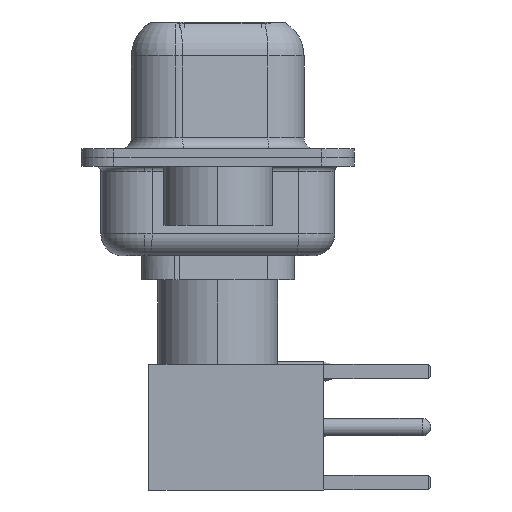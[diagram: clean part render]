
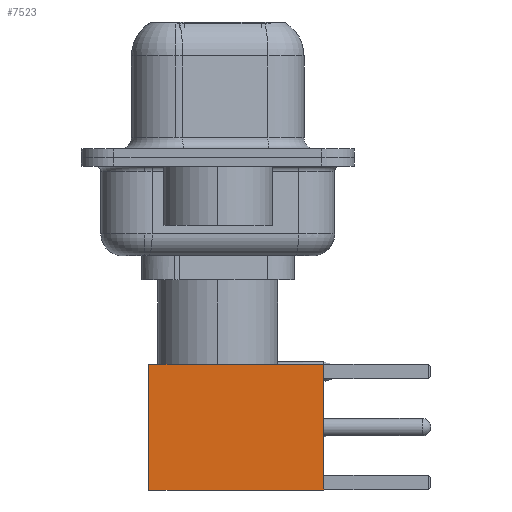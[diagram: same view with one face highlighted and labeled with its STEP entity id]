
A CAD part, left-side view. The second image highlights one B-rep face of the part: STEP entity #7523.
In plain terms, the highlighted face is planar.
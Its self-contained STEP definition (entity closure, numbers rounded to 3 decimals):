
#844 = CARTESIAN_POINT ( 'NONE',  ( -2.875, 2.875, 0. ) ) ;
#2040 = EDGE_CURVE ( 'NONE', #3056, #16021, #9995, .T. ) ;
#2336 = VERTEX_POINT ( 'NONE', #9125 ) ;
#2946 = PLANE ( 'NONE',  #22086 ) ;
#3056 = VERTEX_POINT ( 'NONE', #12006 ) ;
#3095 = LINE ( 'NONE', #12608, #9337 ) ;
#3867 = DIRECTION ( 'NONE',  ( -1., 0., 0. ) ) ;
#4305 = FACE_OUTER_BOUND ( 'NONE', #21728, .T. ) ;
#4921 = ORIENTED_EDGE ( 'NONE', *, *, #8052, .F. ) ;
#5228 = ORIENTED_EDGE ( 'NONE', *, *, #20506, .T. ) ;
#7199 = EDGE_CURVE ( 'NONE', #2336, #10379, #3095, .T. ) ;
#7523 = ADVANCED_FACE ( 'NONE', ( #4305 ), #2946, .T. ) ;
#8052 = EDGE_CURVE ( 'NONE', #2336, #3056, #12764, .T. ) ;
#9125 = CARTESIAN_POINT ( 'NONE',  ( 2.875, 2.875, 8. ) ) ;
#9154 = ORIENTED_EDGE ( 'NONE', *, *, #7199, .T. ) ;
#9337 = VECTOR ( 'NONE', #10874, 1000. ) ;
#9995 = LINE ( 'NONE', #10241, #19126 ) ;
#10241 = CARTESIAN_POINT ( 'NONE',  ( -2.875, 2.875, 0. ) ) ;
#10379 = VERTEX_POINT ( 'NONE', #16181 ) ;
#10874 = DIRECTION ( 'NONE',  ( 0., 0., -1. ) ) ;
#11281 = CARTESIAN_POINT ( 'NONE',  ( 0., 2.875, 0. ) ) ;
#12006 = CARTESIAN_POINT ( 'NONE',  ( -2.875, 2.875, 8. ) ) ;
#12340 = CARTESIAN_POINT ( 'NONE',  ( 2.875, 2.875, 0. ) ) ;
#12608 = CARTESIAN_POINT ( 'NONE',  ( 2.875, 2.875, 0. ) ) ;
#12764 = LINE ( 'NONE', #14883, #22501 ) ;
#14883 = CARTESIAN_POINT ( 'NONE',  ( 0., 2.875, 8. ) ) ;
#15005 = DIRECTION ( 'NONE',  ( -1., 0., 0. ) ) ;
#15679 = DIRECTION ( 'NONE',  ( 0., 0., -1. ) ) ;
#16021 = VERTEX_POINT ( 'NONE', #844 ) ;
#16181 = CARTESIAN_POINT ( 'NONE',  ( 2.875, 2.875, 0. ) ) ;
#17903 = DIRECTION ( 'NONE',  ( 0., 0., 1. ) ) ;
#18252 = VECTOR ( 'NONE', #3867, 1000. ) ;
#19126 = VECTOR ( 'NONE', #15679, 1000. ) ;
#20506 = EDGE_CURVE ( 'NONE', #10379, #16021, #24261, .T. ) ;
#21499 = DIRECTION ( 'NONE',  ( 0., 1., 0. ) ) ;
#21728 = EDGE_LOOP ( 'NONE', ( #9154, #5228, #23799, #4921 ) ) ;
#22086 = AXIS2_PLACEMENT_3D ( 'NONE', #12340, #21499, #17903 ) ;
#22501 = VECTOR ( 'NONE', #15005, 1000. ) ;
#23799 = ORIENTED_EDGE ( 'NONE', *, *, #2040, .F. ) ;
#24261 = LINE ( 'NONE', #11281, #18252 ) ;
